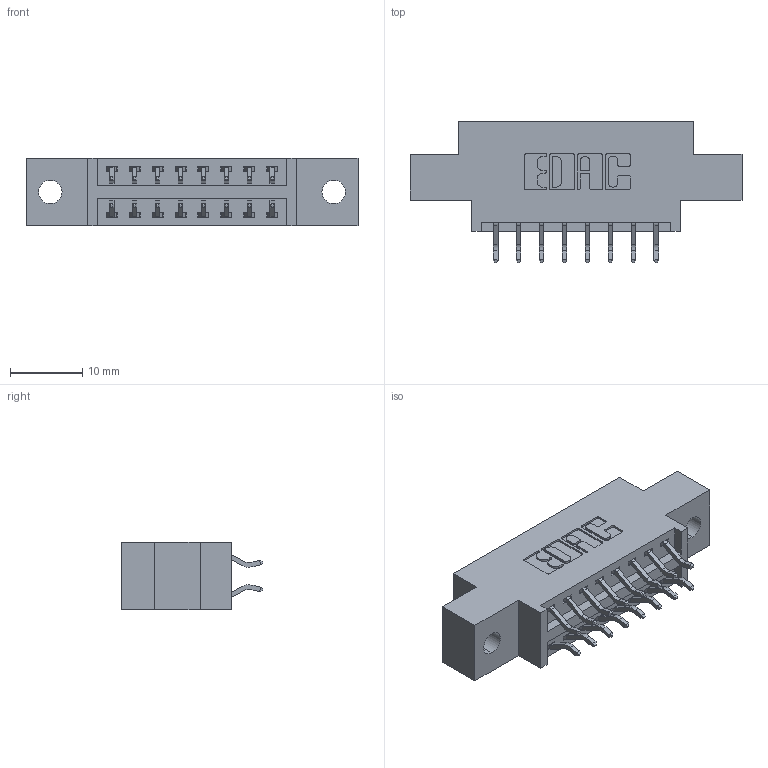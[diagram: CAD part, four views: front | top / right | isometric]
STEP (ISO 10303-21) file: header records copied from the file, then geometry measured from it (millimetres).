
FILE_DESCRIPTION (( 'STEP AP203' ), '1' );
FILE_NAME ('346-016-556-802.STEP', '2022-05-18T16:16:43', ( '' ), ( '' ), 'SwSTEP 2.0', 'SolidWorks 2020', '' );
FILE_SCHEMA (( 'CONFIG_CONTROL_DESIGN' ));
Length unit declared in the file: inch
Products named in the file (3): 345-292-001_556 Tail; 346 Part_0.170 Offset - 0.128 Dia; 346-016-556-802
Assembly tree (17 placements, depth 2):
  346-016-556-802
    346 Part_0.170 Offset - 0.128 Dia
    345-292-001_556 Tail  x16
Bounding box: 45.97 x 19.57 x 9.4 mm (x, y, z)
Volume: 4027 mm3; surface area: 4896.5 mm2
Topology: 17 solids, 17 shells, 1054 faces, 3109 edges, 2050 vertices
Faces by surface type: plane 704, cylinder 350
Entity records: 10153 total; most frequent: CARTESIAN_POINT 1736, ORIENTED_EDGE 1658, DIRECTION 1569, EDGE_CURVE 829, LINE 657, VECTOR 657, VERTEX_POINT 550, AXIS2_PLACEMENT_3D 456
